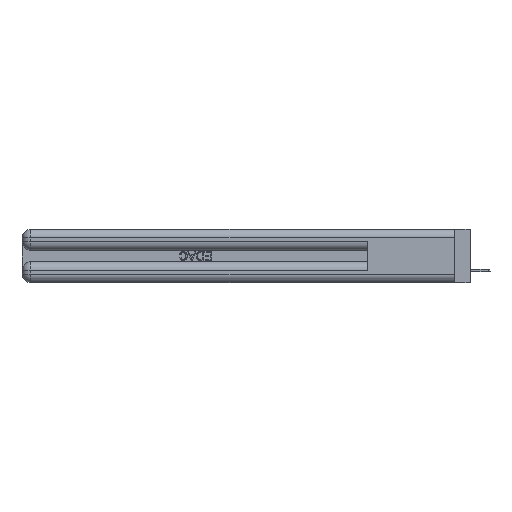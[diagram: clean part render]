
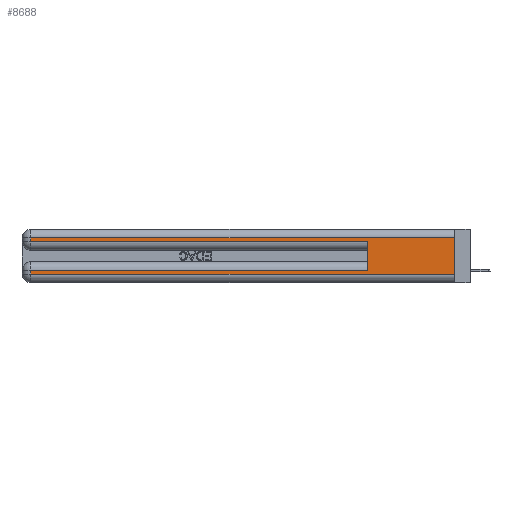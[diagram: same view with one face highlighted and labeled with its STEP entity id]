
A CAD part, left-side view. The second image highlights one B-rep face of the part: STEP entity #8688.
In plain terms, the highlighted planar face has unit normal (-1, 0, 0).
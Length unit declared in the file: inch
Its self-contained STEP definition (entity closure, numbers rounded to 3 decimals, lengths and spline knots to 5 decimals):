
#1065 = CARTESIAN_POINT ( 'NONE',  ( 0., 2.94, 0.31 ) ) ;
#1113 = LINE ( 'NONE', #40177, #3689 ) ;
#1149 = VERTEX_POINT ( 'NONE', #1065 ) ;
#1478 = LINE ( 'NONE', #22969, #29597 ) ;
#1715 = ORIENTED_EDGE ( 'NONE', *, *, #29393, .T. ) ;
#1807 = EDGE_CURVE ( 'NONE', #1149, #42729, #3732, .T. ) ;
#2480 = VECTOR ( 'NONE', #35795, 39.37008 ) ;
#2794 = CARTESIAN_POINT ( 'NONE',  ( 0., 2.94, 0.37 ) ) ;
#2855 = DIRECTION ( 'NONE',  ( 0., -1., 0. ) ) ;
#3269 = CARTESIAN_POINT ( 'NONE',  ( 0., 2.94, 0.37 ) ) ;
#3689 = VECTOR ( 'NONE', #11730, 39.37008 ) ;
#3732 = LINE ( 'NONE', #3269, #5345 ) ;
#5345 = VECTOR ( 'NONE', #17849, 39.37008 ) ;
#5862 = CARTESIAN_POINT ( 'NONE',  ( 0., 0., 0.285 ) ) ;
#6648 = DIRECTION ( 'NONE',  ( 0., 0., -1. ) ) ;
#7247 = VERTEX_POINT ( 'NONE', #17972 ) ;
#7563 = LINE ( 'NONE', #21698, #2480 ) ;
#8688 = ADVANCED_FACE ( 'NONE', ( #12825 ), #16751, .F. ) ;
#9645 = LINE ( 'NONE', #37635, #32621 ) ;
#10034 = CARTESIAN_POINT ( 'NONE',  ( 0., 0., 0.37 ) ) ;
#10618 = ORIENTED_EDGE ( 'NONE', *, *, #30139, .F. ) ;
#11730 = DIRECTION ( 'NONE',  ( 0., 1., 0. ) ) ;
#12825 = FACE_OUTER_BOUND ( 'NONE', #38015, .T. ) ;
#14293 = CARTESIAN_POINT ( 'NONE',  ( 0., 2.94, 0.06 ) ) ;
#14464 = VECTOR ( 'NONE', #24298, 39.37008 ) ;
#14770 = VERTEX_POINT ( 'NONE', #19107 ) ;
#14787 = VECTOR ( 'NONE', #6648, 39.37008 ) ;
#16565 = AXIS2_PLACEMENT_3D ( 'NONE', #10034, #41035, #30410 ) ;
#16693 = VERTEX_POINT ( 'NONE', #33332 ) ;
#16751 = PLANE ( 'NONE',  #16565 ) ;
#17849 = DIRECTION ( 'NONE',  ( 0., 0., -1. ) ) ;
#17972 = CARTESIAN_POINT ( 'NONE',  ( 0., 0.6, 0.085 ) ) ;
#19107 = CARTESIAN_POINT ( 'NONE',  ( 0., 2.94, 0.085 ) ) ;
#19730 = DIRECTION ( 'NONE',  ( 0., 0., 1. ) ) ;
#20844 = ORIENTED_EDGE ( 'NONE', *, *, #1807, .T. ) ;
#20945 = VECTOR ( 'NONE', #2855, 39.37008 ) ;
#21698 = CARTESIAN_POINT ( 'NONE',  ( 0., 0., 0.06 ) ) ;
#22969 = CARTESIAN_POINT ( 'NONE',  ( 0., 0.6, 0.145 ) ) ;
#23236 = EDGE_CURVE ( 'NONE', #14770, #32503, #31475, .T. ) ;
#24298 = DIRECTION ( 'NONE',  ( 0., 0., -1. ) ) ;
#25968 = ORIENTED_EDGE ( 'NONE', *, *, #23236, .T. ) ;
#27931 = EDGE_CURVE ( 'NONE', #42794, #31699, #31889, .T. ) ;
#29393 = EDGE_CURVE ( 'NONE', #42794, #1149, #1113, .T. ) ;
#29597 = VECTOR ( 'NONE', #19730, 39.37008 ) ;
#30139 = EDGE_CURVE ( 'NONE', #7247, #16693, #1478, .T. ) ;
#30410 = DIRECTION ( 'NONE',  ( 0., 0., -1. ) ) ;
#30860 = ORIENTED_EDGE ( 'NONE', *, *, #34157, .T. ) ;
#30945 = CARTESIAN_POINT ( 'NONE',  ( 0., 0., 0.37 ) ) ;
#30999 = EDGE_CURVE ( 'NONE', #7247, #14770, #9645, .T. ) ;
#31040 = CARTESIAN_POINT ( 'NONE',  ( 0., 0., 0.31 ) ) ;
#31475 = LINE ( 'NONE', #2794, #14464 ) ;
#31699 = VERTEX_POINT ( 'NONE', #40724 ) ;
#31889 = LINE ( 'NONE', #30945, #14787 ) ;
#32080 = ORIENTED_EDGE ( 'NONE', *, *, #36205, .T. ) ;
#32503 = VERTEX_POINT ( 'NONE', #14293 ) ;
#32621 = VECTOR ( 'NONE', #38093, 39.37008 ) ;
#33332 = CARTESIAN_POINT ( 'NONE',  ( 0., 0.6, 0.285 ) ) ;
#34157 = EDGE_CURVE ( 'NONE', #32503, #31699, #7563, .T. ) ;
#35795 = DIRECTION ( 'NONE',  ( 0., -1., 0. ) ) ;
#36205 = EDGE_CURVE ( 'NONE', #42729, #16693, #41012, .T. ) ;
#36235 = ORIENTED_EDGE ( 'NONE', *, *, #30999, .T. ) ;
#37635 = CARTESIAN_POINT ( 'NONE',  ( 0., 0., 0.085 ) ) ;
#38015 = EDGE_LOOP ( 'NONE', ( #40176, #1715, #20844, #32080, #10618, #36235, #25968, #30860 ) ) ;
#38093 = DIRECTION ( 'NONE',  ( 0., 1., 0. ) ) ;
#40176 = ORIENTED_EDGE ( 'NONE', *, *, #27931, .F. ) ;
#40177 = CARTESIAN_POINT ( 'NONE',  ( 0., 0., 0.31 ) ) ;
#40724 = CARTESIAN_POINT ( 'NONE',  ( 0., 0., 0.06 ) ) ;
#40766 = CARTESIAN_POINT ( 'NONE',  ( 0., 2.94, 0.285 ) ) ;
#41012 = LINE ( 'NONE', #5862, #20945 ) ;
#41035 = DIRECTION ( 'NONE',  ( 1., 0., 0. ) ) ;
#42729 = VERTEX_POINT ( 'NONE', #40766 ) ;
#42794 = VERTEX_POINT ( 'NONE', #31040 ) ;
